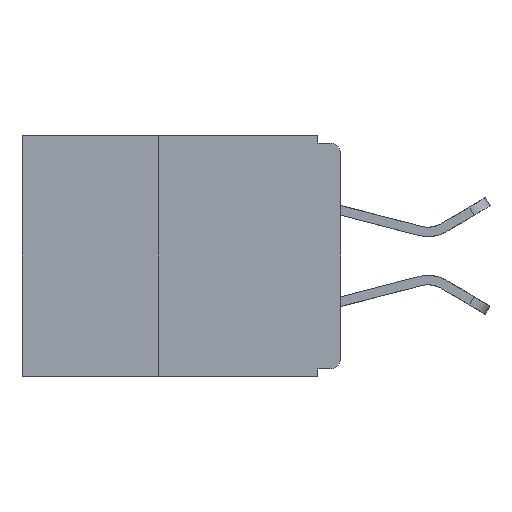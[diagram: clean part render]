
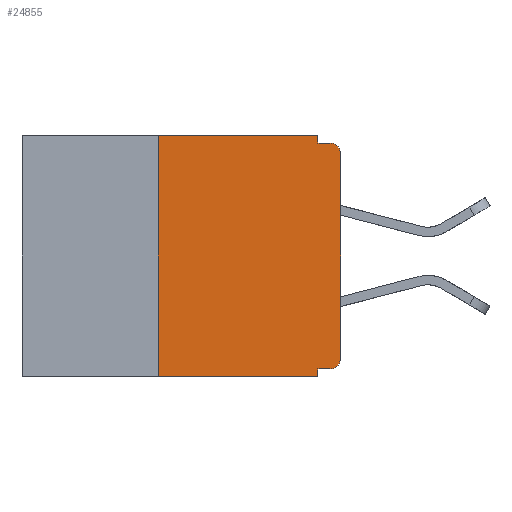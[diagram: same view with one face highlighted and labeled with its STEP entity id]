
A CAD part, left-side view. The second image highlights one B-rep face of the part: STEP entity #24855.
In plain terms, the highlighted planar face has unit normal (-1, 0, 0).
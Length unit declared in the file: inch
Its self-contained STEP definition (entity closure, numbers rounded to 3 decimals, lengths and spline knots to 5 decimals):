
#467 = ORIENTED_EDGE ( 'NONE', *, *, #7008, .F. ) ;
#834 = LINE ( 'NONE', #11937, #2379 ) ;
#991 = CARTESIAN_POINT ( 'NONE',  ( 0., 0.25, -0.33 ) ) ;
#1022 = FACE_OUTER_BOUND ( 'NONE', #27817, .T. ) ;
#1767 = LINE ( 'NONE', #17570, #14239 ) ;
#2369 = ORIENTED_EDGE ( 'NONE', *, *, #22212, .T. ) ;
#2375 = DIRECTION ( 'NONE',  ( 0., -1., 0. ) ) ;
#2379 = VECTOR ( 'NONE', #11895, 39.37008 ) ;
#2679 = CARTESIAN_POINT ( 'NONE',  ( 0., 0.031, -0.33 ) ) ;
#3329 = LINE ( 'NONE', #24799, #22453 ) ;
#3438 = VERTEX_POINT ( 'NONE', #991 ) ;
#4120 = CARTESIAN_POINT ( 'NONE',  ( 0., 0., -0.32 ) ) ;
#5012 = DIRECTION ( 'NONE',  ( 0., -1., 0. ) ) ;
#5201 = EDGE_CURVE ( 'NONE', #3438, #6359, #15322, .T. ) ;
#5653 = ORIENTED_EDGE ( 'NONE', *, *, #8113, .T. ) ;
#6359 = VERTEX_POINT ( 'NONE', #22801 ) ;
#6945 = VERTEX_POINT ( 'NONE', #13035 ) ;
#6995 = VERTEX_POINT ( 'NONE', #12158 ) ;
#7008 = EDGE_CURVE ( 'NONE', #24724, #6995, #834, .T. ) ;
#7571 = DIRECTION ( 'NONE',  ( 0., 0., -1. ) ) ;
#8113 = EDGE_CURVE ( 'NONE', #6945, #14797, #26785, .T. ) ;
#8286 = LINE ( 'NONE', #22514, #14151 ) ;
#8578 = CARTESIAN_POINT ( 'NONE',  ( 0., 0.015, -0.025 ) ) ;
#8657 = ORIENTED_EDGE ( 'NONE', *, *, #24186, .F. ) ;
#8813 = LINE ( 'NONE', #4120, #14701 ) ;
#8832 = LINE ( 'NONE', #14989, #21356 ) ;
#9173 = PLANE ( 'NONE',  #10158 ) ;
#9833 = CARTESIAN_POINT ( 'NONE',  ( 0., 0.437, 0. ) ) ;
#9983 = DIRECTION ( 'NONE',  ( -1., 0., 0. ) ) ;
#10158 = AXIS2_PLACEMENT_3D ( 'NONE', #26588, #29041, #14229 ) ;
#10215 = CARTESIAN_POINT ( 'NONE',  ( 0., 0.015, -0.01 ) ) ;
#11067 = DIRECTION ( 'NONE',  ( 0., 0., -1. ) ) ;
#11128 = ORIENTED_EDGE ( 'NONE', *, *, #17621, .T. ) ;
#11895 = DIRECTION ( 'NONE',  ( 0., 0., -1. ) ) ;
#11937 = CARTESIAN_POINT ( 'NONE',  ( 0., 0.031, 0. ) ) ;
#12158 = CARTESIAN_POINT ( 'NONE',  ( 0., 0.031, -0.01 ) ) ;
#12595 = VERTEX_POINT ( 'NONE', #2679 ) ;
#12669 = ORIENTED_EDGE ( 'NONE', *, *, #30172, .T. ) ;
#13035 = CARTESIAN_POINT ( 'NONE',  ( 0., 0.015, -0.32 ) ) ;
#14151 = VECTOR ( 'NONE', #7571, 39.37008 ) ;
#14229 = DIRECTION ( 'NONE',  ( 0., 0., -1. ) ) ;
#14239 = VECTOR ( 'NONE', #29844, 39.37008 ) ;
#14442 = AXIS2_PLACEMENT_3D ( 'NONE', #8578, #25986, #11067 ) ;
#14701 = VECTOR ( 'NONE', #16593, 39.37008 ) ;
#14797 = VERTEX_POINT ( 'NONE', #24243 ) ;
#14907 = EDGE_CURVE ( 'NONE', #6359, #24724, #16539, .T. ) ;
#14951 = EDGE_CURVE ( 'NONE', #15267, #12595, #8286, .T. ) ;
#14989 = CARTESIAN_POINT ( 'NONE',  ( 0., 0.437, -0.33 ) ) ;
#15267 = VERTEX_POINT ( 'NONE', #16318 ) ;
#15322 = LINE ( 'NONE', #29435, #21180 ) ;
#16318 = CARTESIAN_POINT ( 'NONE',  ( 0., 0.031, -0.32 ) ) ;
#16370 = VERTEX_POINT ( 'NONE', #30141 ) ;
#16539 = LINE ( 'NONE', #9833, #28110 ) ;
#16593 = DIRECTION ( 'NONE',  ( 0., 1., 0. ) ) ;
#17570 = CARTESIAN_POINT ( 'NONE',  ( 0., 0., 0. ) ) ;
#17621 = EDGE_CURVE ( 'NONE', #3438, #12595, #8832, .T. ) ;
#18734 = EDGE_CURVE ( 'NONE', #6995, #31457, #3329, .T. ) ;
#20395 = ORIENTED_EDGE ( 'NONE', *, *, #14907, .F. ) ;
#20733 = ORIENTED_EDGE ( 'NONE', *, *, #5201, .F. ) ;
#21180 = VECTOR ( 'NONE', #28902, 39.37008 ) ;
#21356 = VECTOR ( 'NONE', #5012, 39.37008 ) ;
#21373 = ORIENTED_EDGE ( 'NONE', *, *, #14951, .F. ) ;
#22212 = EDGE_CURVE ( 'NONE', #16370, #31457, #25290, .T. ) ;
#22453 = VECTOR ( 'NONE', #2375, 39.37008 ) ;
#22514 = CARTESIAN_POINT ( 'NONE',  ( 0., 0.031, -0.33 ) ) ;
#22801 = CARTESIAN_POINT ( 'NONE',  ( 0., 0.25, 0. ) ) ;
#23722 = AXIS2_PLACEMENT_3D ( 'NONE', #24941, #9983, #27369 ) ;
#24186 = EDGE_CURVE ( 'NONE', #6945, #15267, #8813, .T. ) ;
#24243 = CARTESIAN_POINT ( 'NONE',  ( 0., 0., -0.305 ) ) ;
#24724 = VERTEX_POINT ( 'NONE', #26056 ) ;
#24799 = CARTESIAN_POINT ( 'NONE',  ( 0., 0., -0.01 ) ) ;
#24855 = ADVANCED_FACE ( 'NONE', ( #1022 ), #9173, .F. ) ;
#24941 = CARTESIAN_POINT ( 'NONE',  ( 0., 0.015, -0.305 ) ) ;
#25290 = CIRCLE ( 'NONE', #14442, 0.015 ) ;
#25986 = DIRECTION ( 'NONE',  ( -1., 0., 0. ) ) ;
#26056 = CARTESIAN_POINT ( 'NONE',  ( 0., 0.031, 0. ) ) ;
#26588 = CARTESIAN_POINT ( 'NONE',  ( 0., 0.437, 0. ) ) ;
#26785 = CIRCLE ( 'NONE', #23722, 0.015 ) ;
#27369 = DIRECTION ( 'NONE',  ( 0., 0., -1. ) ) ;
#27817 = EDGE_LOOP ( 'NONE', ( #12669, #2369, #28175, #467, #20395, #20733, #11128, #21373, #8657, #5653 ) ) ;
#28110 = VECTOR ( 'NONE', #29687, 39.37008 ) ;
#28175 = ORIENTED_EDGE ( 'NONE', *, *, #18734, .F. ) ;
#28902 = DIRECTION ( 'NONE',  ( 0., 0., 1. ) ) ;
#29041 = DIRECTION ( 'NONE',  ( 1., 0., 0. ) ) ;
#29435 = CARTESIAN_POINT ( 'NONE',  ( 0., 0.25, -0.33 ) ) ;
#29687 = DIRECTION ( 'NONE',  ( 0., -1., 0. ) ) ;
#29844 = DIRECTION ( 'NONE',  ( 0., 0., 1. ) ) ;
#30141 = CARTESIAN_POINT ( 'NONE',  ( 0., 0., -0.025 ) ) ;
#30172 = EDGE_CURVE ( 'NONE', #14797, #16370, #1767, .T. ) ;
#31457 = VERTEX_POINT ( 'NONE', #10215 ) ;
